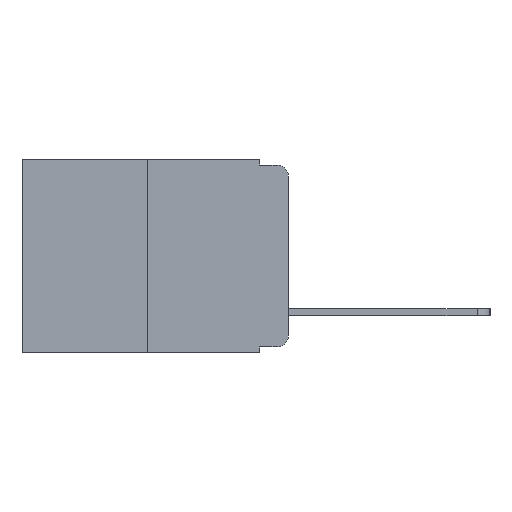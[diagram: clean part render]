
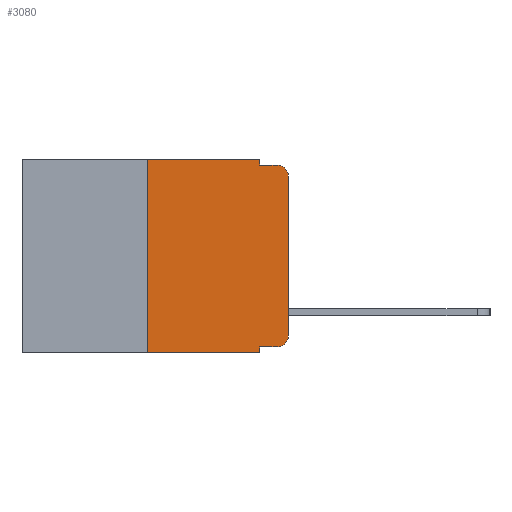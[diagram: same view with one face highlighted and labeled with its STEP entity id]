
A CAD part, left-side view. The second image highlights one B-rep face of the part: STEP entity #3080.
In plain terms, the highlighted planar face has unit normal (-1, 0, 0).
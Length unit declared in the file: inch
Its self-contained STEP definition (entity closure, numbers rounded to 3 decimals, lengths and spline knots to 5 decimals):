
#48 = DIRECTION ( 'NONE',  ( 0., 0., -1. ) ) ;
#61 = CIRCLE ( 'NONE', #3022, 0.02 ) ;
#78 = EDGE_CURVE ( 'NONE', #10037, #7839, #6935, .T. ) ;
#146 = CARTESIAN_POINT ( 'NONE',  ( 0., 0.051, -0.01 ) ) ;
#238 = VERTEX_POINT ( 'NONE', #10650 ) ;
#433 = CARTESIAN_POINT ( 'NONE',  ( 0., 0.473, 0. ) ) ;
#671 = CARTESIAN_POINT ( 'NONE',  ( 0., 0.02, -0.313 ) ) ;
#712 = DIRECTION ( 'NONE',  ( 0., 0., -1. ) ) ;
#845 = CARTESIAN_POINT ( 'NONE',  ( 0., 0.02, -0.03 ) ) ;
#944 = DIRECTION ( 'NONE',  ( -1., 0., 0. ) ) ;
#1038 = EDGE_CURVE ( 'NONE', #4013, #10017, #8744, .T. ) ;
#1098 = EDGE_CURVE ( 'NONE', #11233, #1571, #13140, .T. ) ;
#1137 = LINE ( 'NONE', #7498, #3062 ) ;
#1571 = VERTEX_POINT ( 'NONE', #1939 ) ;
#1819 = DIRECTION ( 'NONE',  ( 0., 0., -1. ) ) ;
#1939 = CARTESIAN_POINT ( 'NONE',  ( 0., 0.02, -0.333 ) ) ;
#2262 = EDGE_CURVE ( 'NONE', #10037, #238, #1137, .T. ) ;
#2288 = EDGE_CURVE ( 'NONE', #2464, #3862, #61, .T. ) ;
#2464 = VERTEX_POINT ( 'NONE', #3799 ) ;
#3013 = VECTOR ( 'NONE', #12117, 39.37008 ) ;
#3022 = AXIS2_PLACEMENT_3D ( 'NONE', #845, #944, #712 ) ;
#3062 = VECTOR ( 'NONE', #12197, 39.37008 ) ;
#3080 = ADVANCED_FACE ( 'NONE', ( #6715 ), #10782, .F. ) ;
#3210 = LINE ( 'NONE', #433, #6356 ) ;
#3520 = CARTESIAN_POINT ( 'NONE',  ( 0., 0.051, -0.333 ) ) ;
#3717 = CARTESIAN_POINT ( 'NONE',  ( 0., 0.051, -0.333 ) ) ;
#3799 = CARTESIAN_POINT ( 'NONE',  ( 0., 0., -0.03 ) ) ;
#3862 = VERTEX_POINT ( 'NONE', #4655 ) ;
#4013 = VERTEX_POINT ( 'NONE', #7139 ) ;
#4241 = DIRECTION ( 'NONE',  ( 0., -1., 0. ) ) ;
#4655 = CARTESIAN_POINT ( 'NONE',  ( 0., 0.02, -0.01 ) ) ;
#5082 = CARTESIAN_POINT ( 'NONE',  ( 0., 0., 0. ) ) ;
#5332 = EDGE_LOOP ( 'NONE', ( #5641, #6061, #6731, #7404, #7442, #8177, #8222, #8444, #8533, #8619 ) ) ;
#5641 = ORIENTED_EDGE ( 'NONE', *, *, #7596, .T. ) ;
#5668 = EDGE_CURVE ( 'NONE', #10017, #3862, #6585, .T. ) ;
#5943 = CARTESIAN_POINT ( 'NONE',  ( 0., 0.051, 0. ) ) ;
#6008 = VECTOR ( 'NONE', #48, 39.37008 ) ;
#6061 = ORIENTED_EDGE ( 'NONE', *, *, #2288, .T. ) ;
#6186 = DIRECTION ( 'NONE',  ( 0., -1., 0. ) ) ;
#6356 = VECTOR ( 'NONE', #6186, 39.37008 ) ;
#6397 = CARTESIAN_POINT ( 'NONE',  ( 0., 0.051, 0. ) ) ;
#6585 = LINE ( 'NONE', #146, #11444 ) ;
#6715 = FACE_OUTER_BOUND ( 'NONE', #5332, .T. ) ;
#6731 = ORIENTED_EDGE ( 'NONE', *, *, #5668, .F. ) ;
#6774 = EDGE_CURVE ( 'NONE', #238, #4013, #3210, .T. ) ;
#6818 = CARTESIAN_POINT ( 'NONE',  ( 0., 0.051, -0.343 ) ) ;
#6935 = LINE ( 'NONE', #8090, #11740 ) ;
#7139 = CARTESIAN_POINT ( 'NONE',  ( 0., 0.051, 0. ) ) ;
#7404 = ORIENTED_EDGE ( 'NONE', *, *, #1038, .F. ) ;
#7442 = ORIENTED_EDGE ( 'NONE', *, *, #6774, .F. ) ;
#7498 = CARTESIAN_POINT ( 'NONE',  ( 0., 0.25, 0. ) ) ;
#7596 = EDGE_CURVE ( 'NONE', #8293, #2464, #8837, .T. ) ;
#7839 = VERTEX_POINT ( 'NONE', #6818 ) ;
#7949 = VECTOR ( 'NONE', #9038, 39.37008 ) ;
#8090 = CARTESIAN_POINT ( 'NONE',  ( 0., 0.473, -0.343 ) ) ;
#8177 = ORIENTED_EDGE ( 'NONE', *, *, #2262, .F. ) ;
#8222 = ORIENTED_EDGE ( 'NONE', *, *, #78, .T. ) ;
#8293 = VERTEX_POINT ( 'NONE', #10270 ) ;
#8444 = ORIENTED_EDGE ( 'NONE', *, *, #12903, .F. ) ;
#8446 = DIRECTION ( 'NONE',  ( -1., 0., 0. ) ) ;
#8533 = ORIENTED_EDGE ( 'NONE', *, *, #1098, .T. ) ;
#8619 = ORIENTED_EDGE ( 'NONE', *, *, #9431, .T. ) ;
#8744 = LINE ( 'NONE', #6397, #6008 ) ;
#8837 = LINE ( 'NONE', #5082, #3013 ) ;
#9038 = DIRECTION ( 'NONE',  ( 0., 0., -1. ) ) ;
#9303 = DIRECTION ( 'NONE',  ( 0., -1., 0. ) ) ;
#9431 = EDGE_CURVE ( 'NONE', #1571, #8293, #10157, .T. ) ;
#10017 = VERTEX_POINT ( 'NONE', #10989 ) ;
#10037 = VERTEX_POINT ( 'NONE', #11934 ) ;
#10157 = CIRCLE ( 'NONE', #11566, 0.02 ) ;
#10270 = CARTESIAN_POINT ( 'NONE',  ( 0., 0., -0.313 ) ) ;
#10650 = CARTESIAN_POINT ( 'NONE',  ( 0., 0.25, 0. ) ) ;
#10697 = DIRECTION ( 'NONE',  ( 0., 0., -1. ) ) ;
#10701 = VECTOR ( 'NONE', #4241, 39.37008 ) ;
#10715 = DIRECTION ( 'NONE',  ( 1., 0., 0. ) ) ;
#10782 = PLANE ( 'NONE',  #13288 ) ;
#10919 = CARTESIAN_POINT ( 'NONE',  ( 0., 0.473, 0. ) ) ;
#10989 = CARTESIAN_POINT ( 'NONE',  ( 0., 0.051, -0.01 ) ) ;
#11233 = VERTEX_POINT ( 'NONE', #3520 ) ;
#11444 = VECTOR ( 'NONE', #13423, 39.37008 ) ;
#11566 = AXIS2_PLACEMENT_3D ( 'NONE', #671, #8446, #1819 ) ;
#11740 = VECTOR ( 'NONE', #9303, 39.37008 ) ;
#11934 = CARTESIAN_POINT ( 'NONE',  ( 0., 0.25, -0.343 ) ) ;
#12117 = DIRECTION ( 'NONE',  ( 0., 0., 1. ) ) ;
#12197 = DIRECTION ( 'NONE',  ( 0., 0., 1. ) ) ;
#12903 = EDGE_CURVE ( 'NONE', #11233, #7839, #12986, .T. ) ;
#12986 = LINE ( 'NONE', #5943, #7949 ) ;
#13140 = LINE ( 'NONE', #3717, #10701 ) ;
#13288 = AXIS2_PLACEMENT_3D ( 'NONE', #10919, #10715, #10697 ) ;
#13423 = DIRECTION ( 'NONE',  ( 0., -1., 0. ) ) ;
